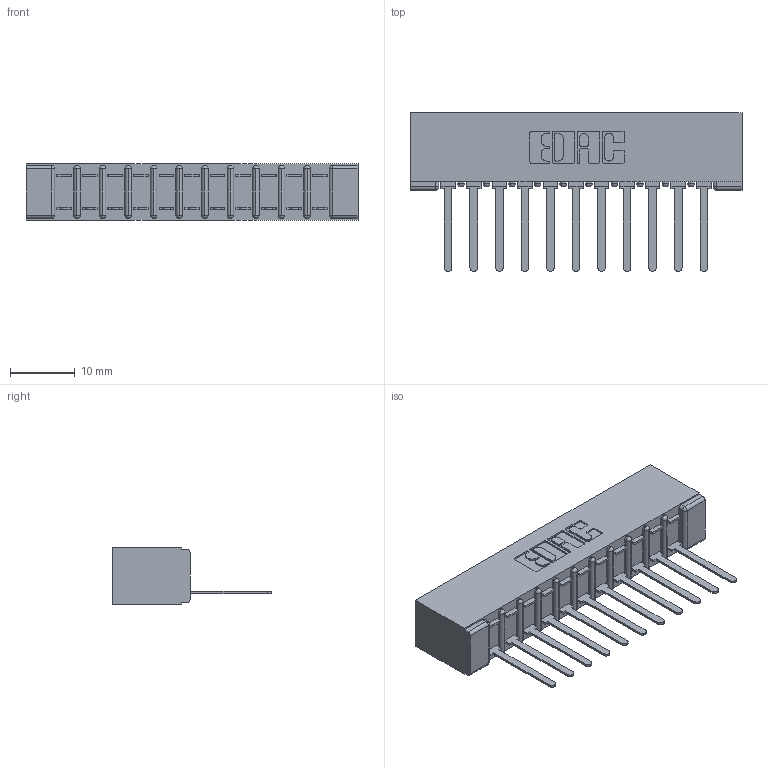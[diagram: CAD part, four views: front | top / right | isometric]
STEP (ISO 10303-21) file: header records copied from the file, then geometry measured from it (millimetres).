
FILE_DESCRIPTION (( 'STEP AP203' ), '1' );
FILE_NAME ('357-011-441-101.STEP', '2020-09-30T10:02:48', ( '' ), ( '' ), 'SwSTEP 2.0', 'SolidWorks 2020', '' );
FILE_SCHEMA (( 'CONFIG_CONTROL_DESIGN' ));
Length unit declared in the file: inch
Products named in the file (3): 307 Part_No Mounting Lugs; 357-011-441-101; 307-290-002_541
Assembly tree (12 placements, depth 2):
  357-011-441-101
    307 Part_No Mounting Lugs
    307-290-002_541  x11
Bounding box: 51.46 x 24.59 x 8.71 mm (x, y, z)
Volume: 3664.9 mm3; surface area: 6748.9 mm2
Topology: 12 solids, 12 shells, 936 faces, 2851 edges, 1866 vertices
Faces by surface type: plane 561, cylinder 351, sphere 24
Entity records: 13692 total; most frequent: CARTESIAN_POINT 2304, ORIENTED_EDGE 2294, DIRECTION 2251, EDGE_CURVE 1147, LINE 865, VECTOR 865, VERTEX_POINT 746, AXIS2_PLACEMENT_3D 693
